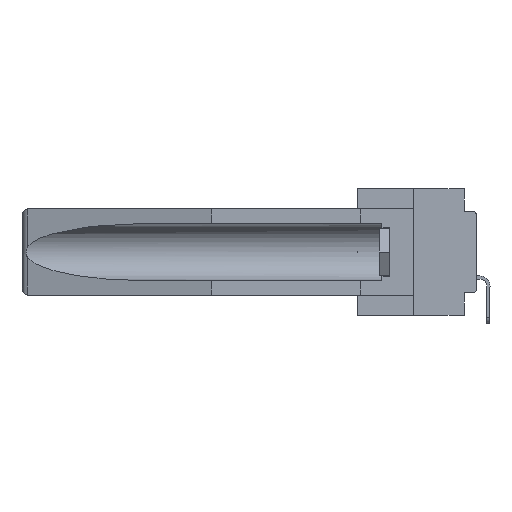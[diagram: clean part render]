
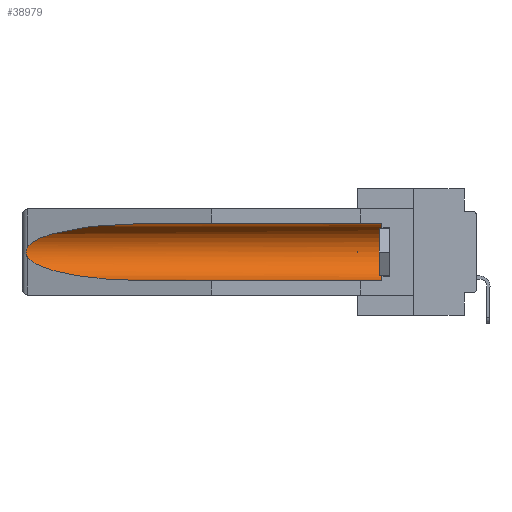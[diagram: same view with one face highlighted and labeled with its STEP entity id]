
A CAD part, left-side view. The second image highlights one B-rep face of the part: STEP entity #38979.
In plain terms, the highlighted cylindrical face has radius 2.857 mm (diameter 5.715 mm), a partial arc.
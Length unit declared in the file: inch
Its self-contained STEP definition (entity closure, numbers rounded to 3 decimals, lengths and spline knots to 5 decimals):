
#548 = VERTEX_POINT ( 'NONE', #975 ) ;
#975 = CARTESIAN_POINT ( 'NONE',  ( 0.155, 0.126, -0.284 ) ) ;
#1201 = CARTESIAN_POINT ( 'NONE',  ( 0.26597, 1.52961, -0.15275 ) ) ;
#2033 = CARTESIAN_POINT ( 'NONE',  ( 0.155, 0.126, -0.059 ) ) ;
#2544 = VERTEX_POINT ( 'NONE', #22810 ) ;
#2642 = CARTESIAN_POINT ( 'NONE',  ( 0.26537, 1.52718, -0.14972 ) ) ;
#3352 = DIRECTION ( 'NONE',  ( 0., 1., 0. ) ) ;
#3374 = EDGE_CURVE ( 'NONE', #2544, #24179, #12970, .T. ) ;
#4160 = VECTOR ( 'NONE', #3352, 39.37008 ) ;
#4661 = CARTESIAN_POINT ( 'NONE',  ( 0.2673, 1.53269, -0.17917 ) ) ;
#5518 = CARTESIAN_POINT ( 'NONE',  ( 0.21114, 1.30732, -0.284 ) ) ;
#5851 = CARTESIAN_POINT ( 'NONE',  ( 0.25451, 1.48313, -0.09465 ) ) ;
#5919 = B_SPLINE_CURVE_WITH_KNOTS ( 'NONE', 3,
 ( #16726, #1201, #22789, #28655, #10497, #37897, #4661, #7716, #25468, #22933 ),
 .UNSPECIFIED., .F., .F.,
 ( 4, 2, 2, 2, 4 ),
 ( 0., 0.00029, 0.00058, 0.00087, 0.00117 ),
 .UNSPECIFIED. ) ;
#6294 = ORIENTED_EDGE ( 'NONE', *, *, #29683, .F. ) ;
#7716 = CARTESIAN_POINT ( 'NONE',  ( 0.26655, 1.53094, -0.18657 ) ) ;
#8284 = DIRECTION ( 'NONE',  ( 0., 0., 1. ) ) ;
#8433 = LINE ( 'NONE', #33484, #4160 ) ;
#8491 = EDGE_CURVE ( 'NONE', #16177, #2544, #5919, .T. ) ;
#8663 = CARTESIAN_POINT ( 'NONE',  ( 0.155, -0.30754, -0.1715 ) ) ;
#8682 = CARTESIAN_POINT ( 'NONE',  ( 0.155, 1.07973, -0.284 ) ) ;
#10164 = EDGE_CURVE ( 'NONE', #34726, #16177, #13461, .T. ) ;
#10497 = CARTESIAN_POINT ( 'NONE',  ( 0.2675, 1.53308, -0.16763 ) ) ;
#12970 =( BOUNDED_CURVE ( )  B_SPLINE_CURVE ( 3, ( #20348, #14774, #5518, #8682 ),
 .UNSPECIFIED., .F., .F. ) 
 B_SPLINE_CURVE_WITH_KNOTS ( ( 4, 4 ),
 ( 0.1948, 1.5708 ),
 .UNSPECIFIED. ) 
 CURVE ( )  GEOMETRIC_REPRESENTATION_ITEM ( )  RATIONAL_B_SPLINE_CURVE ( ( 1., 0.848, 0.848, 1. ) ) 
 REPRESENTATION_ITEM ( '' )  );
#13461 =( BOUNDED_CURVE ( )  B_SPLINE_CURVE ( 3, ( #38164, #39214, #5851, #2642 ),
 .UNSPECIFIED., .F., .F. ) 
 B_SPLINE_CURVE_WITH_KNOTS ( ( 4, 4 ),
 ( 4.71239, 6.08839 ),
 .UNSPECIFIED. ) 
 CURVE ( )  GEOMETRIC_REPRESENTATION_ITEM ( )  RATIONAL_B_SPLINE_CURVE ( ( 1., 0.848, 0.848, 1. ) ) 
 REPRESENTATION_ITEM ( '' )  );
#14097 = VERTEX_POINT ( 'NONE', #2033 ) ;
#14436 = CARTESIAN_POINT ( 'NONE',  ( 0.26537, 1.52718, -0.14972 ) ) ;
#14774 = CARTESIAN_POINT ( 'NONE',  ( 0.25451, 1.48313, -0.24835 ) ) ;
#16177 = VERTEX_POINT ( 'NONE', #14436 ) ;
#16726 = CARTESIAN_POINT ( 'NONE',  ( 0.26537, 1.52718, -0.14972 ) ) ;
#16728 = ORIENTED_EDGE ( 'NONE', *, *, #3374, .T. ) ;
#17160 = DIRECTION ( 'NONE',  ( 0., 1., 0. ) ) ;
#18822 = FACE_OUTER_BOUND ( 'NONE', #30847, .T. ) ;
#20348 = CARTESIAN_POINT ( 'NONE',  ( 0.26537, 1.52718, -0.19328 ) ) ;
#20865 = CIRCLE ( 'NONE', #31821, 0.1125 ) ;
#21757 = ORIENTED_EDGE ( 'NONE', *, *, #8491, .T. ) ;
#22789 = CARTESIAN_POINT ( 'NONE',  ( 0.26654, 1.53092, -0.15636 ) ) ;
#22810 = CARTESIAN_POINT ( 'NONE',  ( 0.26537, 1.52718, -0.19328 ) ) ;
#22933 = CARTESIAN_POINT ( 'NONE',  ( 0.26537, 1.52718, -0.19328 ) ) ;
#24179 = VERTEX_POINT ( 'NONE', #28129 ) ;
#25468 = CARTESIAN_POINT ( 'NONE',  ( 0.26597, 1.5296, -0.19026 ) ) ;
#25793 = EDGE_CURVE ( 'NONE', #14097, #34726, #28946, .T. ) ;
#26041 = CARTESIAN_POINT ( 'NONE',  ( 0.155, -0.30754, -0.059 ) ) ;
#28129 = CARTESIAN_POINT ( 'NONE',  ( 0.155, 1.07973, -0.284 ) ) ;
#28535 = ORIENTED_EDGE ( 'NONE', *, *, #10164, .T. ) ;
#28655 = CARTESIAN_POINT ( 'NONE',  ( 0.2673, 1.5327, -0.16383 ) ) ;
#28946 = LINE ( 'NONE', #26041, #29413 ) ;
#29413 = VECTOR ( 'NONE', #17160, 39.37008 ) ;
#29683 = EDGE_CURVE ( 'NONE', #548, #24179, #8433, .T. ) ;
#30847 = EDGE_LOOP ( 'NONE', ( #28535, #21757, #16728, #6294, #38856, #35588 ) ) ;
#31821 = AXIS2_PLACEMENT_3D ( 'NONE', #38114, #38248, #32575 ) ;
#32575 = DIRECTION ( 'NONE',  ( 0., 0., 1. ) ) ;
#32973 = AXIS2_PLACEMENT_3D ( 'NONE', #8663, #35862, #8284 ) ;
#33484 = CARTESIAN_POINT ( 'NONE',  ( 0.155, -0.30754, -0.284 ) ) ;
#34726 = VERTEX_POINT ( 'NONE', #36997 ) ;
#35588 = ORIENTED_EDGE ( 'NONE', *, *, #25793, .T. ) ;
#35862 = DIRECTION ( 'NONE',  ( 0., 1., 0. ) ) ;
#36145 = EDGE_CURVE ( 'NONE', #548, #14097, #20865, .T. ) ;
#36830 = CYLINDRICAL_SURFACE ( 'NONE', #32973, 0.1125 ) ;
#36997 = CARTESIAN_POINT ( 'NONE',  ( 0.155, 1.07973, -0.059 ) ) ;
#37897 = CARTESIAN_POINT ( 'NONE',  ( 0.2675, 1.53308, -0.17534 ) ) ;
#38114 = CARTESIAN_POINT ( 'NONE',  ( 0.155, 0.126, -0.1715 ) ) ;
#38164 = CARTESIAN_POINT ( 'NONE',  ( 0.155, 1.07973, -0.059 ) ) ;
#38248 = DIRECTION ( 'NONE',  ( 0., -1., 0. ) ) ;
#38856 = ORIENTED_EDGE ( 'NONE', *, *, #36145, .T. ) ;
#38979 = ADVANCED_FACE ( 'NONE', ( #18822 ), #36830, .F. ) ;
#39214 = CARTESIAN_POINT ( 'NONE',  ( 0.21114, 1.30732, -0.059 ) ) ;
